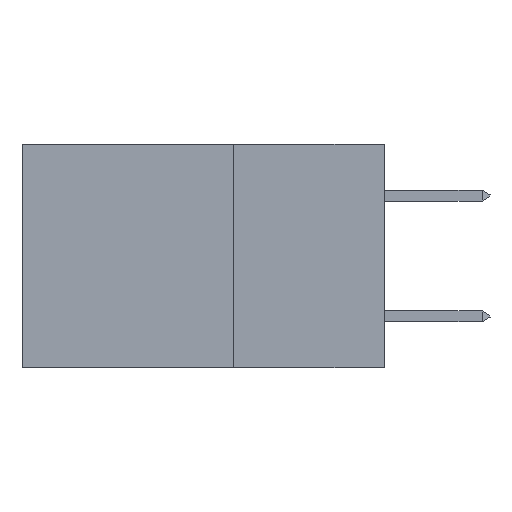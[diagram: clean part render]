
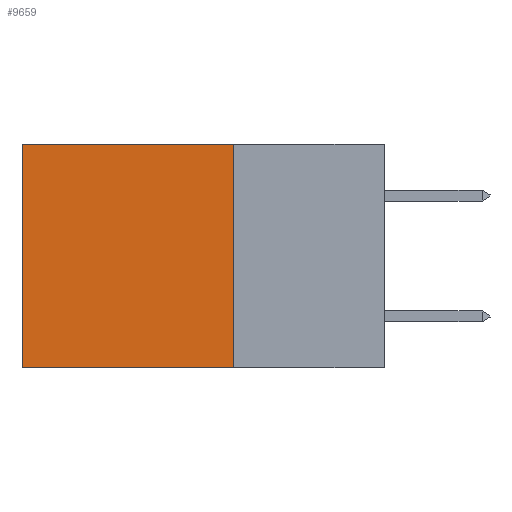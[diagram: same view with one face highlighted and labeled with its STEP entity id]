
A CAD part, left-side view. The second image highlights one B-rep face of the part: STEP entity #9659.
In plain terms, the highlighted planar face has unit normal (-1, 0, 0).
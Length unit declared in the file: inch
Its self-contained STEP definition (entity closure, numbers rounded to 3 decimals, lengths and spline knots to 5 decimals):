
#3099 = EDGE_CURVE ( 'NONE', #19546, #15945, #26302, .T. ) ;
#4822 = VECTOR ( 'NONE', #37505, 39.37008 ) ;
#5254 = DIRECTION ( 'NONE',  ( 0., 0., -1. ) ) ;
#6487 = DIRECTION ( 'NONE',  ( 0., 0., -1. ) ) ;
#6880 = CARTESIAN_POINT ( 'NONE',  ( 0.2875, 0.25, 0. ) ) ;
#7797 = CARTESIAN_POINT ( 'NONE',  ( 0.2875, 0.25, 0. ) ) ;
#8779 = EDGE_CURVE ( 'NONE', #40979, #33451, #40309, .T. ) ;
#9659 = ADVANCED_FACE ( 'NONE', ( #39219 ), #39658, .F. ) ;
#10219 = VECTOR ( 'NONE', #40937, 39.37008 ) ;
#12429 = AXIS2_PLACEMENT_3D ( 'NONE', #7797, #40058, #5254 ) ;
#14698 = VECTOR ( 'NONE', #22903, 39.37008 ) ;
#15036 = ORIENTED_EDGE ( 'NONE', *, *, #22433, .T. ) ;
#15257 = CARTESIAN_POINT ( 'NONE',  ( 0.2875, 0.25, -0.37 ) ) ;
#15945 = VERTEX_POINT ( 'NONE', #38152 ) ;
#19546 = VERTEX_POINT ( 'NONE', #26919 ) ;
#20524 = ORIENTED_EDGE ( 'NONE', *, *, #8779, .T. ) ;
#20765 = ORIENTED_EDGE ( 'NONE', *, *, #3099, .F. ) ;
#20832 = ORIENTED_EDGE ( 'NONE', *, *, #38300, .F. ) ;
#21616 = CARTESIAN_POINT ( 'NONE',  ( 0.2875, 0.25, 0. ) ) ;
#22433 = EDGE_CURVE ( 'NONE', #33451, #15945, #36100, .T. ) ;
#22903 = DIRECTION ( 'NONE',  ( 0., 1., 0. ) ) ;
#26302 = LINE ( 'NONE', #15257, #10219 ) ;
#26919 = CARTESIAN_POINT ( 'NONE',  ( 0.2875, 0.25, -0.37 ) ) ;
#27550 = VECTOR ( 'NONE', #6487, 39.37008 ) ;
#30488 = LINE ( 'NONE', #21616, #4822 ) ;
#33451 = VERTEX_POINT ( 'NONE', #35770 ) ;
#35770 = CARTESIAN_POINT ( 'NONE',  ( 0.2875, 0.6, 0. ) ) ;
#36100 = LINE ( 'NONE', #38226, #27550 ) ;
#37505 = DIRECTION ( 'NONE',  ( 0., 0., -1. ) ) ;
#38152 = CARTESIAN_POINT ( 'NONE',  ( 0.2875, 0.6, -0.37 ) ) ;
#38226 = CARTESIAN_POINT ( 'NONE',  ( 0.2875, 0.6, 0. ) ) ;
#38300 = EDGE_CURVE ( 'NONE', #40979, #19546, #30488, .T. ) ;
#39219 = FACE_OUTER_BOUND ( 'NONE', #39578, .T. ) ;
#39578 = EDGE_LOOP ( 'NONE', ( #15036, #20765, #20832, #20524 ) ) ;
#39658 = PLANE ( 'NONE',  #12429 ) ;
#40058 = DIRECTION ( 'NONE',  ( 1., 0., 0. ) ) ;
#40309 = LINE ( 'NONE', #6880, #14698 ) ;
#40937 = DIRECTION ( 'NONE',  ( 0., 1., 0. ) ) ;
#40979 = VERTEX_POINT ( 'NONE', #41463 ) ;
#41463 = CARTESIAN_POINT ( 'NONE',  ( 0.2875, 0.25, 0. ) ) ;
